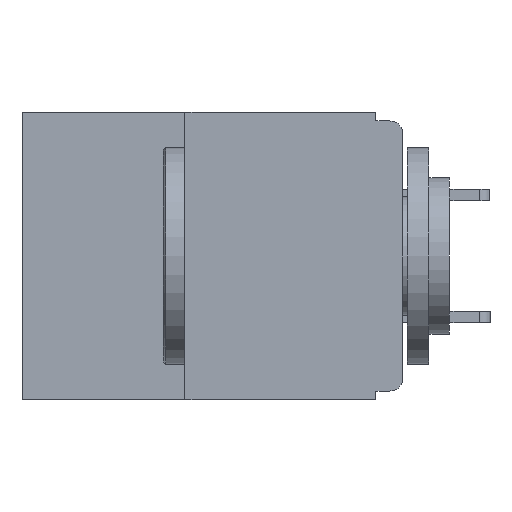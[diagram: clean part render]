
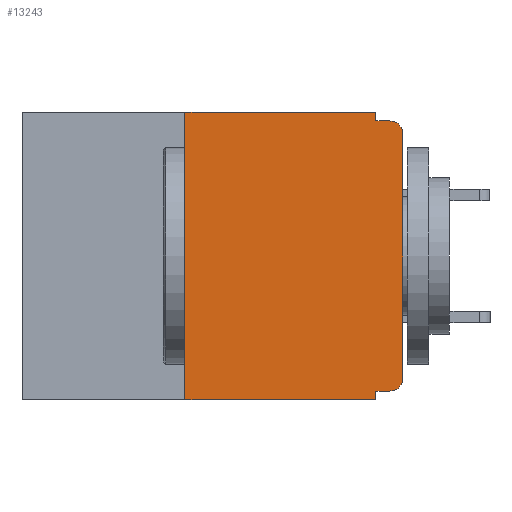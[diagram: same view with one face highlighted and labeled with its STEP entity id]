
A CAD part, left-side view. The second image highlights one B-rep face of the part: STEP entity #13243.
In plain terms, the highlighted planar face has unit normal (-1, 0, 0).
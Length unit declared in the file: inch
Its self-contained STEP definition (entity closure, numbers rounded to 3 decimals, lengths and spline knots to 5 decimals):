
#159 = EDGE_CURVE ( 'NONE', #11946, #5208, #10561, .T. ) ;
#283 = ORIENTED_EDGE ( 'NONE', *, *, #9263, .F. ) ;
#606 = DIRECTION ( 'NONE',  ( -1., 0., 0. ) ) ;
#618 = LINE ( 'NONE', #1059, #11640 ) ;
#770 = EDGE_LOOP ( 'NONE', ( #3896, #15878, #5274, #5737, #6691, #14808, #7617, #283, #12409, #5058 ) ) ;
#835 = DIRECTION ( 'NONE',  ( 0., -1., 0. ) ) ;
#866 = LINE ( 'NONE', #16248, #16192 ) ;
#1053 = VERTEX_POINT ( 'NONE', #14822 ) ;
#1059 = CARTESIAN_POINT ( 'NONE',  ( 0., 0., -0.01 ) ) ;
#1298 = PLANE ( 'NONE',  #11711 ) ;
#1359 = LINE ( 'NONE', #11060, #4743 ) ;
#1513 = CARTESIAN_POINT ( 'NONE',  ( 0., 0., 0. ) ) ;
#1791 = AXIS2_PLACEMENT_3D ( 'NONE', #5091, #606, #3126 ) ;
#1796 = DIRECTION ( 'NONE',  ( 0., 0., -1. ) ) ;
#2550 = DIRECTION ( 'NONE',  ( 0., -1., 0. ) ) ;
#2770 = DIRECTION ( 'NONE',  ( 1., 0., 0. ) ) ;
#2786 = EDGE_CURVE ( 'NONE', #17111, #16669, #5191, .T. ) ;
#2796 = DIRECTION ( 'NONE',  ( 0., 1., 0. ) ) ;
#3126 = DIRECTION ( 'NONE',  ( 0., 0., -1. ) ) ;
#3403 = CARTESIAN_POINT ( 'NONE',  ( 0., 0.031, 0. ) ) ;
#3407 = DIRECTION ( 'NONE',  ( 0., 0., -1. ) ) ;
#3791 = VERTEX_POINT ( 'NONE', #3403 ) ;
#3848 = CARTESIAN_POINT ( 'NONE',  ( 0., 0.015, -0.025 ) ) ;
#3896 = ORIENTED_EDGE ( 'NONE', *, *, #16368, .T. ) ;
#4332 = EDGE_CURVE ( 'NONE', #1053, #10219, #12913, .T. ) ;
#4743 = VECTOR ( 'NONE', #835, 39.37008 ) ;
#4957 = VECTOR ( 'NONE', #1796, 39.37008 ) ;
#5058 = ORIENTED_EDGE ( 'NONE', *, *, #2786, .T. ) ;
#5090 = VERTEX_POINT ( 'NONE', #13043 ) ;
#5091 = CARTESIAN_POINT ( 'NONE',  ( 0., 0.015, -0.305 ) ) ;
#5191 = CIRCLE ( 'NONE', #1791, 0.015 ) ;
#5208 = VERTEX_POINT ( 'NONE', #11792 ) ;
#5274 = ORIENTED_EDGE ( 'NONE', *, *, #9522, .F. ) ;
#5524 = EDGE_CURVE ( 'NONE', #10219, #3791, #15481, .T. ) ;
#5589 = CARTESIAN_POINT ( 'NONE',  ( 0., 0.437, 0. ) ) ;
#5737 = ORIENTED_EDGE ( 'NONE', *, *, #15796, .F. ) ;
#5767 = CARTESIAN_POINT ( 'NONE',  ( 0., 0.031, -0.01 ) ) ;
#5962 = CARTESIAN_POINT ( 'NONE',  ( 0., 0.031, -0.32 ) ) ;
#6007 = AXIS2_PLACEMENT_3D ( 'NONE', #3848, #14648, #3407 ) ;
#6109 = VECTOR ( 'NONE', #11715, 39.37008 ) ;
#6572 = CARTESIAN_POINT ( 'NONE',  ( 0., 0., -0.305 ) ) ;
#6685 = FACE_OUTER_BOUND ( 'NONE', #770, .T. ) ;
#6691 = ORIENTED_EDGE ( 'NONE', *, *, #5524, .F. ) ;
#7092 = VECTOR ( 'NONE', #2796, 39.37008 ) ;
#7331 = VERTEX_POINT ( 'NONE', #5962 ) ;
#7617 = ORIENTED_EDGE ( 'NONE', *, *, #8794, .T. ) ;
#7735 = EDGE_CURVE ( 'NONE', #17111, #7331, #10995, .T. ) ;
#8178 = DIRECTION ( 'NONE',  ( 0., 0., 1. ) ) ;
#8362 = DIRECTION ( 'NONE',  ( 0., -1., 0. ) ) ;
#8422 = CARTESIAN_POINT ( 'NONE',  ( 0., 0.437, 0. ) ) ;
#8714 = CARTESIAN_POINT ( 'NONE',  ( 0., 0.25, 0. ) ) ;
#8794 = EDGE_CURVE ( 'NONE', #1053, #5090, #1359, .T. ) ;
#9092 = VERTEX_POINT ( 'NONE', #5767 ) ;
#9176 = DIRECTION ( 'NONE',  ( 0., 0., -1. ) ) ;
#9263 = EDGE_CURVE ( 'NONE', #7331, #5090, #866, .T. ) ;
#9522 = EDGE_CURVE ( 'NONE', #9092, #5208, #618, .T. ) ;
#10219 = VERTEX_POINT ( 'NONE', #8714 ) ;
#10232 = CARTESIAN_POINT ( 'NONE',  ( 0., 0.25, -0.33 ) ) ;
#10561 = CIRCLE ( 'NONE', #6007, 0.015 ) ;
#10995 = LINE ( 'NONE', #12974, #7092 ) ;
#11060 = CARTESIAN_POINT ( 'NONE',  ( 0., 0.437, -0.33 ) ) ;
#11640 = VECTOR ( 'NONE', #2550, 39.37008 ) ;
#11711 = AXIS2_PLACEMENT_3D ( 'NONE', #5589, #2770, #12945 ) ;
#11715 = DIRECTION ( 'NONE',  ( 0., 0., 1. ) ) ;
#11768 = VECTOR ( 'NONE', #8362, 39.37008 ) ;
#11792 = CARTESIAN_POINT ( 'NONE',  ( 0., 0.015, -0.01 ) ) ;
#11946 = VERTEX_POINT ( 'NONE', #18231 ) ;
#11999 = CARTESIAN_POINT ( 'NONE',  ( 0., 0.031, 0. ) ) ;
#12409 = ORIENTED_EDGE ( 'NONE', *, *, #7735, .F. ) ;
#12913 = LINE ( 'NONE', #10232, #16155 ) ;
#12945 = DIRECTION ( 'NONE',  ( 0., 0., -1. ) ) ;
#12974 = CARTESIAN_POINT ( 'NONE',  ( 0., 0., -0.32 ) ) ;
#13043 = CARTESIAN_POINT ( 'NONE',  ( 0., 0.031, -0.33 ) ) ;
#13243 = ADVANCED_FACE ( 'NONE', ( #6685 ), #1298, .F. ) ;
#14648 = DIRECTION ( 'NONE',  ( -1., 0., 0. ) ) ;
#14808 = ORIENTED_EDGE ( 'NONE', *, *, #4332, .F. ) ;
#14822 = CARTESIAN_POINT ( 'NONE',  ( 0., 0.25, -0.33 ) ) ;
#15481 = LINE ( 'NONE', #8422, #11768 ) ;
#15796 = EDGE_CURVE ( 'NONE', #3791, #9092, #16003, .T. ) ;
#15878 = ORIENTED_EDGE ( 'NONE', *, *, #159, .T. ) ;
#16003 = LINE ( 'NONE', #11999, #4957 ) ;
#16155 = VECTOR ( 'NONE', #8178, 39.37008 ) ;
#16192 = VECTOR ( 'NONE', #9176, 39.37008 ) ;
#16248 = CARTESIAN_POINT ( 'NONE',  ( 0., 0.031, -0.33 ) ) ;
#16368 = EDGE_CURVE ( 'NONE', #16669, #11946, #17445, .T. ) ;
#16415 = CARTESIAN_POINT ( 'NONE',  ( 0., 0.015, -0.32 ) ) ;
#16669 = VERTEX_POINT ( 'NONE', #6572 ) ;
#17111 = VERTEX_POINT ( 'NONE', #16415 ) ;
#17445 = LINE ( 'NONE', #1513, #6109 ) ;
#18231 = CARTESIAN_POINT ( 'NONE',  ( 0., 0., -0.025 ) ) ;
